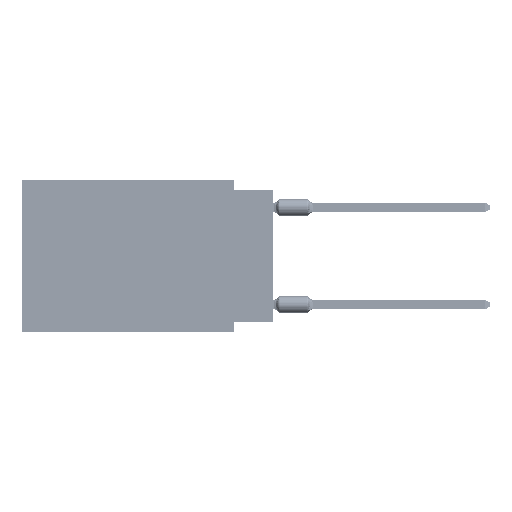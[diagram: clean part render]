
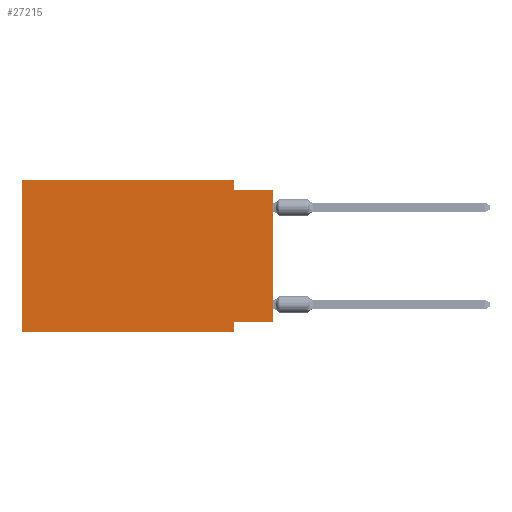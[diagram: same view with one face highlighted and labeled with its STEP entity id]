
A CAD part, left-side view. The second image highlights one B-rep face of the part: STEP entity #27215.
In plain terms, the highlighted planar face has unit normal (-1, 0, 0).
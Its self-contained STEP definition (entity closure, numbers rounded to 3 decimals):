
#137 = CARTESIAN_POINT ( 'NONE',  ( 0., 0., -9.271 ) ) ;
#1839 = CARTESIAN_POINT ( 'NONE',  ( 0., 0., -0.635 ) ) ;
#2224 = LINE ( 'NONE', #1839, #44642 ) ;
#4372 = ORIENTED_EDGE ( 'NONE', *, *, #25968, .F. ) ;
#8442 = LINE ( 'NONE', #51870, #37243 ) ;
#9194 = DIRECTION ( 'NONE',  ( 0., 0., -1. ) ) ;
#9281 = CARTESIAN_POINT ( 'NONE',  ( 0., 2.54, -9.906 ) ) ;
#10596 = CARTESIAN_POINT ( 'NONE',  ( 0., 0., 0. ) ) ;
#11342 = VERTEX_POINT ( 'NONE', #55188 ) ;
#12993 = LINE ( 'NONE', #74004, #47062 ) ;
#13777 = DIRECTION ( 'NONE',  ( 0., -1., 0. ) ) ;
#14167 = CARTESIAN_POINT ( 'NONE',  ( 0., 16.383, -9.906 ) ) ;
#14813 = DIRECTION ( 'NONE',  ( 0., -1., 0. ) ) ;
#14922 = VECTOR ( 'NONE', #9194, 1000. ) ;
#16130 = LINE ( 'NONE', #53563, #72701 ) ;
#16738 = VERTEX_POINT ( 'NONE', #28285 ) ;
#16924 = PLANE ( 'NONE',  #32076 ) ;
#20778 = VERTEX_POINT ( 'NONE', #74544 ) ;
#22125 = DIRECTION ( 'NONE',  ( 0., 0., -1. ) ) ;
#22952 = LINE ( 'NONE', #10596, #67688 ) ;
#23307 = CARTESIAN_POINT ( 'NONE',  ( 0., 16.383, 0. ) ) ;
#24467 = DIRECTION ( 'NONE',  ( 0., 1., 0. ) ) ;
#25968 = EDGE_CURVE ( 'NONE', #75120, #43520, #16130, .T. ) ;
#27215 = ADVANCED_FACE ( 'NONE', ( #59563 ), #16924, .F. ) ;
#28285 = CARTESIAN_POINT ( 'NONE',  ( 0., 0., -9.271 ) ) ;
#28934 = DIRECTION ( 'NONE',  ( 0., 0., 1. ) ) ;
#29137 = EDGE_CURVE ( 'NONE', #43520, #70898, #12993, .T. ) ;
#30309 = EDGE_LOOP ( 'NONE', ( #43993, #42615, #70680, #78652, #4372, #58035, #73007, #60302 ) ) ;
#30577 = EDGE_CURVE ( 'NONE', #16738, #48987, #54747, .T. ) ;
#32076 = AXIS2_PLACEMENT_3D ( 'NONE', #23307, #47613, #22125 ) ;
#33727 = DIRECTION ( 'NONE',  ( 0., -1., 0. ) ) ;
#33826 = EDGE_CURVE ( 'NONE', #16738, #20778, #22952, .T. ) ;
#37243 = VECTOR ( 'NONE', #14813, 1000. ) ;
#40306 = VECTOR ( 'NONE', #69108, 1000. ) ;
#40320 = EDGE_CURVE ( 'NONE', #48987, #11342, #50746, .T. ) ;
#40768 = EDGE_CURVE ( 'NONE', #70898, #53172, #44683, .T. ) ;
#42615 = ORIENTED_EDGE ( 'NONE', *, *, #55815, .F. ) ;
#43520 = VERTEX_POINT ( 'NONE', #63672 ) ;
#43993 = ORIENTED_EDGE ( 'NONE', *, *, #33826, .T. ) ;
#44642 = VECTOR ( 'NONE', #33727, 1000. ) ;
#44683 = LINE ( 'NONE', #45475, #14922 ) ;
#45475 = CARTESIAN_POINT ( 'NONE',  ( 0., 2.54, 0. ) ) ;
#47062 = VECTOR ( 'NONE', #13777, 1000. ) ;
#47613 = DIRECTION ( 'NONE',  ( 1., 0., 0. ) ) ;
#48987 = VERTEX_POINT ( 'NONE', #50804 ) ;
#49070 = CARTESIAN_POINT ( 'NONE',  ( 0., 2.54, 0. ) ) ;
#50746 = LINE ( 'NONE', #9281, #40306 ) ;
#50804 = CARTESIAN_POINT ( 'NONE',  ( 0., 2.54, -9.271 ) ) ;
#51870 = CARTESIAN_POINT ( 'NONE',  ( 0., 16.383, -9.906 ) ) ;
#53172 = VERTEX_POINT ( 'NONE', #71779 ) ;
#53563 = CARTESIAN_POINT ( 'NONE',  ( 0., 16.383, 0. ) ) ;
#54747 = LINE ( 'NONE', #137, #73889 ) ;
#55188 = CARTESIAN_POINT ( 'NONE',  ( 0., 2.54, -9.906 ) ) ;
#55815 = EDGE_CURVE ( 'NONE', #53172, #20778, #2224, .T. ) ;
#57766 = EDGE_CURVE ( 'NONE', #75120, #11342, #8442, .T. ) ;
#58035 = ORIENTED_EDGE ( 'NONE', *, *, #57766, .T. ) ;
#59563 = FACE_OUTER_BOUND ( 'NONE', #30309, .T. ) ;
#60302 = ORIENTED_EDGE ( 'NONE', *, *, #30577, .F. ) ;
#63672 = CARTESIAN_POINT ( 'NONE',  ( 0., 16.383, 0. ) ) ;
#67688 = VECTOR ( 'NONE', #28934, 1000. ) ;
#69108 = DIRECTION ( 'NONE',  ( 0., 0., -1. ) ) ;
#69960 = DIRECTION ( 'NONE',  ( 0., 0., 1. ) ) ;
#70680 = ORIENTED_EDGE ( 'NONE', *, *, #40768, .F. ) ;
#70898 = VERTEX_POINT ( 'NONE', #49070 ) ;
#71779 = CARTESIAN_POINT ( 'NONE',  ( 0., 2.54, -0.635 ) ) ;
#72701 = VECTOR ( 'NONE', #69960, 1000. ) ;
#73007 = ORIENTED_EDGE ( 'NONE', *, *, #40320, .F. ) ;
#73889 = VECTOR ( 'NONE', #24467, 1000. ) ;
#74004 = CARTESIAN_POINT ( 'NONE',  ( 0., 16.383, 0. ) ) ;
#74544 = CARTESIAN_POINT ( 'NONE',  ( 0., 0., -0.635 ) ) ;
#75120 = VERTEX_POINT ( 'NONE', #14167 ) ;
#78652 = ORIENTED_EDGE ( 'NONE', *, *, #29137, .F. ) ;
